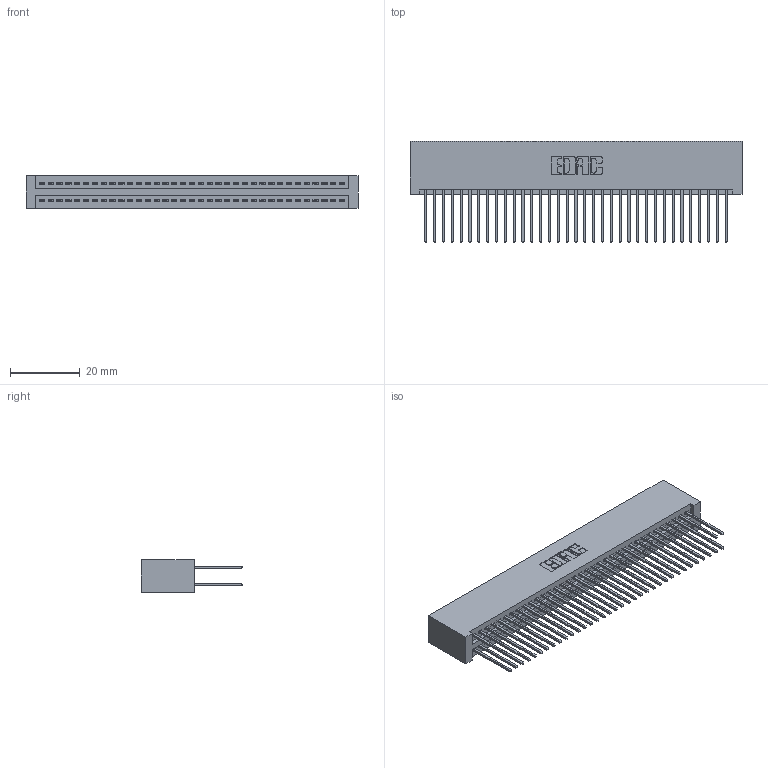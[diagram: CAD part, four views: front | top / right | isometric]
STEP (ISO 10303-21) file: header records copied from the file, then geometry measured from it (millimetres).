
FILE_DESCRIPTION (( 'STEP AP203' ), '1' );
FILE_NAME ('395-070-540-201.STEP', '2018-11-26T18:03:45', ( '' ), ( '' ), 'SwSTEP 2.0', 'SolidWorks 2016', '' );
FILE_SCHEMA (( 'CONFIG_CONTROL_DESIGN' ));
Length unit declared in the file: inch
Products named in the file (3): 345 Part_No Mounting Lugs; 345-292-001_345-293-140; 395-070-540-201
Assembly tree (71 placements, depth 2):
  395-070-540-201
    345 Part_No Mounting Lugs
    345-292-001_345-293-140  x70
Bounding box: 95.5 x 29.13 x 9.4 mm (x, y, z)
Volume: 10093.7 mm3; surface area: 16319 mm2
Topology: 71 solids, 71 shells, 3618 faces, 10747 edges, 7070 vertices
Faces by surface type: plane 2386, cylinder 1232
Entity records: 28145 total; most frequent: CARTESIAN_POINT 4724, ORIENTED_EDGE 4658, DIRECTION 4169, EDGE_CURVE 2329, VECTOR 2065, LINE 2065, VERTEX_POINT 1550, AXIS2_PLACEMENT_3D 1052
